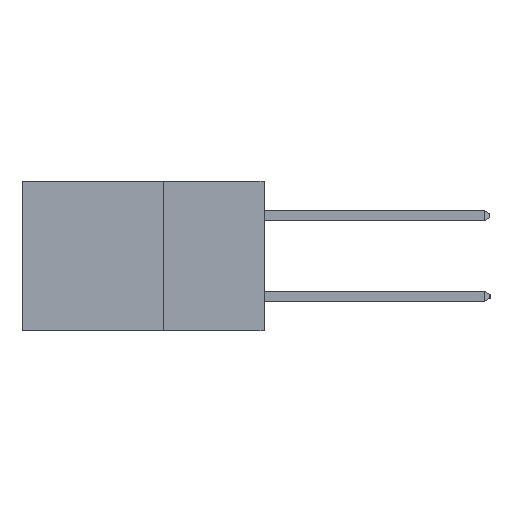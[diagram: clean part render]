
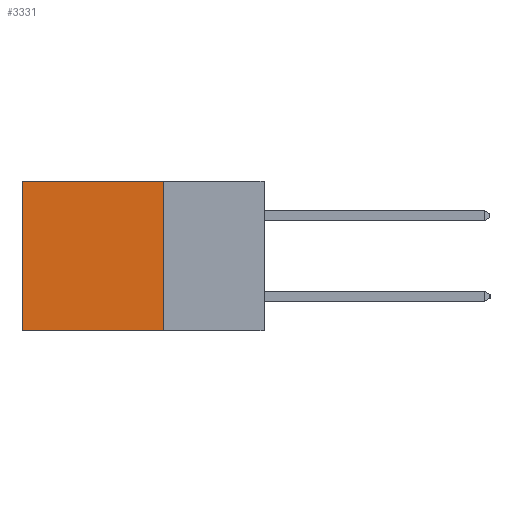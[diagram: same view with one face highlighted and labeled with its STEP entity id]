
A CAD part, left-side view. The second image highlights one B-rep face of the part: STEP entity #3331.
In plain terms, the highlighted planar face has unit normal (-1, 0, 0).
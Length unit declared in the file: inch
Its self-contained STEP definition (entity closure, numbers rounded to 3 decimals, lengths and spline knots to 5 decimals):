
#190 = DIRECTION ( 'NONE',  ( 0., 0., -1. ) ) ;
#383 = DIRECTION ( 'NONE',  ( 1., 0., 0. ) ) ;
#454 = CARTESIAN_POINT ( 'NONE',  ( 0.2615, 0.25, -0.37 ) ) ;
#482 = PLANE ( 'NONE',  #5517 ) ;
#487 = CARTESIAN_POINT ( 'NONE',  ( 0.2615, 0.25, 0. ) ) ;
#801 = VECTOR ( 'NONE', #5575, 39.37008 ) ;
#1372 = VECTOR ( 'NONE', #1637, 39.37008 ) ;
#1559 = VERTEX_POINT ( 'NONE', #18302 ) ;
#1637 = DIRECTION ( 'NONE',  ( 0., 0., -1. ) ) ;
#2181 = ORIENTED_EDGE ( 'NONE', *, *, #5259, .F. ) ;
#2429 = CARTESIAN_POINT ( 'NONE',  ( 0.2615, 0.6, -0.37 ) ) ;
#2511 = LINE ( 'NONE', #10960, #17441 ) ;
#2611 = CARTESIAN_POINT ( 'NONE',  ( 0.2615, 0.25, -0.37 ) ) ;
#3331 = ADVANCED_FACE ( 'NONE', ( #15215 ), #482, .F. ) ;
#3596 = CARTESIAN_POINT ( 'NONE',  ( 0.2615, 0.25, -0.37 ) ) ;
#3881 = ORIENTED_EDGE ( 'NONE', *, *, #8595, .T. ) ;
#4942 = CARTESIAN_POINT ( 'NONE',  ( 0.2615, 0.25, 0. ) ) ;
#5129 = VERTEX_POINT ( 'NONE', #2429 ) ;
#5259 = EDGE_CURVE ( 'NONE', #17385, #5129, #8634, .T. ) ;
#5517 = AXIS2_PLACEMENT_3D ( 'NONE', #454, #383, #190 ) ;
#5575 = DIRECTION ( 'NONE',  ( 0., 1., 0. ) ) ;
#5690 = EDGE_CURVE ( 'NONE', #12695, #1559, #17170, .T. ) ;
#8386 = ORIENTED_EDGE ( 'NONE', *, *, #18291, .F. ) ;
#8595 = EDGE_CURVE ( 'NONE', #1559, #5129, #9179, .T. ) ;
#8634 = LINE ( 'NONE', #2611, #801 ) ;
#9179 = LINE ( 'NONE', #16121, #1372 ) ;
#9293 = DIRECTION ( 'NONE',  ( 0., 1., 0. ) ) ;
#9529 = VECTOR ( 'NONE', #9293, 39.37008 ) ;
#10960 = CARTESIAN_POINT ( 'NONE',  ( 0.2615, 0.25, -0.37 ) ) ;
#12407 = EDGE_LOOP ( 'NONE', ( #3881, #2181, #8386, #15530 ) ) ;
#12417 = DIRECTION ( 'NONE',  ( 0., 0., -1. ) ) ;
#12695 = VERTEX_POINT ( 'NONE', #4942 ) ;
#15215 = FACE_OUTER_BOUND ( 'NONE', #12407, .T. ) ;
#15530 = ORIENTED_EDGE ( 'NONE', *, *, #5690, .T. ) ;
#16121 = CARTESIAN_POINT ( 'NONE',  ( 0.2615, 0.6, -0.37 ) ) ;
#17170 = LINE ( 'NONE', #487, #9529 ) ;
#17385 = VERTEX_POINT ( 'NONE', #3596 ) ;
#17441 = VECTOR ( 'NONE', #12417, 39.37008 ) ;
#18291 = EDGE_CURVE ( 'NONE', #12695, #17385, #2511, .T. ) ;
#18302 = CARTESIAN_POINT ( 'NONE',  ( 0.2615, 0.6, 0. ) ) ;
